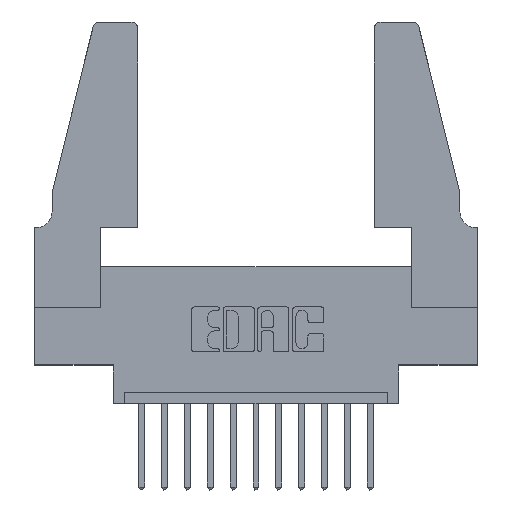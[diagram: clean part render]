
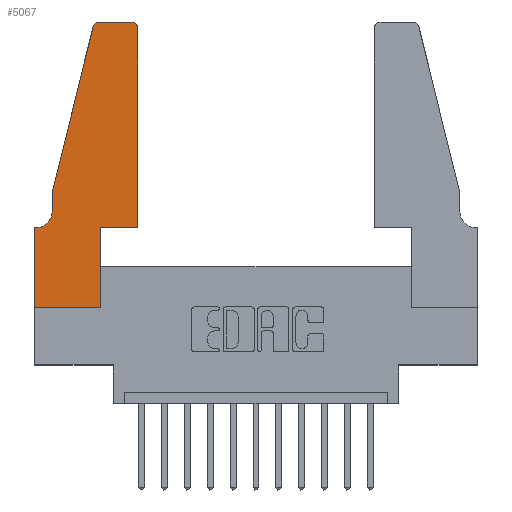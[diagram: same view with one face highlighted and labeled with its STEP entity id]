
A CAD part, top view. The second image highlights one B-rep face of the part: STEP entity #5067.
In plain terms, the highlighted planar face has unit normal (0, 0, 1).
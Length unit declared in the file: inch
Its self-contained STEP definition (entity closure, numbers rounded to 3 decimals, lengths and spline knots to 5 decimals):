
#34 = VECTOR ( 'NONE', #3264, 39.37008 ) ;
#420 = CARTESIAN_POINT ( 'NONE',  ( 0., 0., 0.37 ) ) ;
#542 = ORIENTED_EDGE ( 'NONE', *, *, #3959, .T. ) ;
#629 = EDGE_CURVE ( 'NONE', #13046, #2088, #10502, .T. ) ;
#829 = VERTEX_POINT ( 'NONE', #1325 ) ;
#902 = CARTESIAN_POINT ( 'NONE',  ( 0.0755, 0.5, 0.37 ) ) ;
#965 = VERTEX_POINT ( 'NONE', #14064 ) ;
#1089 = CARTESIAN_POINT ( 'NONE',  ( 0., 0., 0.37 ) ) ;
#1143 = EDGE_CURVE ( 'NONE', #6330, #13046, #6183, .T. ) ;
#1325 = CARTESIAN_POINT ( 'NONE',  ( 0.25487, 1.22718, 0.37 ) ) ;
#1326 = ORIENTED_EDGE ( 'NONE', *, *, #11895, .T. ) ;
#1648 = AXIS2_PLACEMENT_3D ( 'NONE', #6249, #11892, #1726 ) ;
#1726 = DIRECTION ( 'NONE',  ( -1., 0., 0. ) ) ;
#1731 = LINE ( 'NONE', #6070, #8879 ) ;
#2072 = CARTESIAN_POINT ( 'NONE',  ( 0.2605, 1.25, 0.37 ) ) ;
#2088 = VERTEX_POINT ( 'NONE', #2340 ) ;
#2204 = CARTESIAN_POINT ( 'NONE',  ( 0.0755, 0.42, 0.37 ) ) ;
#2340 = CARTESIAN_POINT ( 'NONE',  ( 0.4205, 1.25, 0.37 ) ) ;
#2369 = VERTEX_POINT ( 'NONE', #6469 ) ;
#2382 = CARTESIAN_POINT ( 'NONE',  ( 0.2865, 0.35, 0.37 ) ) ;
#2423 = AXIS2_PLACEMENT_3D ( 'NONE', #4154, #11025, #9827 ) ;
#2503 = DIRECTION ( 'NONE',  ( 1., 0., 0. ) ) ;
#2597 = VERTEX_POINT ( 'NONE', #1089 ) ;
#2632 = VECTOR ( 'NONE', #4961, 39.37008 ) ;
#2845 = LINE ( 'NONE', #13261, #5711 ) ;
#3201 = VERTEX_POINT ( 'NONE', #2204 ) ;
#3264 = DIRECTION ( 'NONE',  ( -1., 0., 0. ) ) ;
#3349 = LINE ( 'NONE', #11802, #2632 ) ;
#3761 = CARTESIAN_POINT ( 'NONE',  ( 0.284, 1.25, 0.37 ) ) ;
#3833 = CARTESIAN_POINT ( 'NONE',  ( 0.4505, 0.35, 0.37 ) ) ;
#3959 = EDGE_CURVE ( 'NONE', #4218, #829, #13787, .T. ) ;
#4154 = CARTESIAN_POINT ( 'NONE',  ( 0.284, 1.22, 0.37 ) ) ;
#4175 = ORIENTED_EDGE ( 'NONE', *, *, #4557, .T. ) ;
#4218 = VERTEX_POINT ( 'NONE', #3761 ) ;
#4557 = EDGE_CURVE ( 'NONE', #2088, #4218, #14088, .T. ) ;
#4961 = DIRECTION ( 'NONE',  ( 0., -1., 0. ) ) ;
#5033 = CARTESIAN_POINT ( 'NONE',  ( 0.0055, 0.35, 0.37 ) ) ;
#5067 = ADVANCED_FACE ( 'NONE', ( #14656 ), #7492, .T. ) ;
#5160 = CARTESIAN_POINT ( 'NONE',  ( 0.4505, 0.35, 0.37 ) ) ;
#5238 = ORIENTED_EDGE ( 'NONE', *, *, #11474, .T. ) ;
#5264 = DIRECTION ( 'NONE',  ( 0., 1., 0. ) ) ;
#5276 = CARTESIAN_POINT ( 'NONE',  ( 0.0755, 0.35, 0.37 ) ) ;
#5323 = DIRECTION ( 'NONE',  ( 0., 0., 1. ) ) ;
#5373 = DIRECTION ( 'NONE',  ( 0., 0., 1. ) ) ;
#5395 = DIRECTION ( 'NONE',  ( -0.239, -0.971, 0. ) ) ;
#5710 = EDGE_CURVE ( 'NONE', #2369, #6330, #2845, .T. ) ;
#5711 = VECTOR ( 'NONE', #14506, 39.37008 ) ;
#6070 = CARTESIAN_POINT ( 'NONE',  ( 0.0755, 0.5, 0.37 ) ) ;
#6183 = LINE ( 'NONE', #5160, #6555 ) ;
#6216 = LINE ( 'NONE', #2382, #13723 ) ;
#6249 = CARTESIAN_POINT ( 'NONE',  ( 0.0055, 0.42, 0.37 ) ) ;
#6330 = VERTEX_POINT ( 'NONE', #3833 ) ;
#6361 = VERTEX_POINT ( 'NONE', #5033 ) ;
#6469 = CARTESIAN_POINT ( 'NONE',  ( 0.2865, 0.35, 0.37 ) ) ;
#6555 = VECTOR ( 'NONE', #5264, 39.37008 ) ;
#6566 = CARTESIAN_POINT ( 'NONE',  ( 0., 0.35, 0.37 ) ) ;
#6747 = EDGE_CURVE ( 'NONE', #965, #2597, #3349, .T. ) ;
#7492 = PLANE ( 'NONE',  #10769 ) ;
#7636 = LINE ( 'NONE', #420, #13898 ) ;
#8405 = ORIENTED_EDGE ( 'NONE', *, *, #14514, .T. ) ;
#8501 = ORIENTED_EDGE ( 'NONE', *, *, #12068, .T. ) ;
#8604 = LINE ( 'NONE', #14433, #10419 ) ;
#8879 = VECTOR ( 'NONE', #13994, 39.37008 ) ;
#9179 = AXIS2_PLACEMENT_3D ( 'NONE', #14462, #5373, #13362 ) ;
#9387 = EDGE_LOOP ( 'NONE', ( #4175, #542, #11279, #14276, #8501, #8405, #9966, #5238, #1326, #11409, #11977, #14247 ) ) ;
#9827 = DIRECTION ( 'NONE',  ( 1., 0., 0. ) ) ;
#9966 = ORIENTED_EDGE ( 'NONE', *, *, #6747, .T. ) ;
#10418 = EDGE_CURVE ( 'NONE', #829, #12775, #8604, .T. ) ;
#10419 = VECTOR ( 'NONE', #5395, 39.37008 ) ;
#10502 = CIRCLE ( 'NONE', #9179, 0.03 ) ;
#10769 = AXIS2_PLACEMENT_3D ( 'NONE', #6566, #5323, #13315 ) ;
#11025 = DIRECTION ( 'NONE',  ( 0., 0., 1. ) ) ;
#11051 = CIRCLE ( 'NONE', #1648, 0.07 ) ;
#11279 = ORIENTED_EDGE ( 'NONE', *, *, #10418, .T. ) ;
#11409 = ORIENTED_EDGE ( 'NONE', *, *, #5710, .T. ) ;
#11474 = EDGE_CURVE ( 'NONE', #2597, #11628, #7636, .T. ) ;
#11628 = VERTEX_POINT ( 'NONE', #11872 ) ;
#11802 = CARTESIAN_POINT ( 'NONE',  ( 0., 0., 0.37 ) ) ;
#11872 = CARTESIAN_POINT ( 'NONE',  ( 0.2865, 0., 0.37 ) ) ;
#11892 = DIRECTION ( 'NONE',  ( 0., 0., -1. ) ) ;
#11895 = EDGE_CURVE ( 'NONE', #11628, #2369, #6216, .T. ) ;
#11977 = ORIENTED_EDGE ( 'NONE', *, *, #1143, .T. ) ;
#12068 = EDGE_CURVE ( 'NONE', #3201, #6361, #11051, .T. ) ;
#12562 = VECTOR ( 'NONE', #14551, 39.37008 ) ;
#12565 = DIRECTION ( 'NONE',  ( 0., 1., 0. ) ) ;
#12571 = EDGE_CURVE ( 'NONE', #12775, #3201, #1731, .T. ) ;
#12775 = VERTEX_POINT ( 'NONE', #902 ) ;
#12826 = CARTESIAN_POINT ( 'NONE',  ( 0.4505, 1.22, 0.37 ) ) ;
#13046 = VERTEX_POINT ( 'NONE', #12826 ) ;
#13261 = CARTESIAN_POINT ( 'NONE',  ( 0.4505, 0.35, 0.37 ) ) ;
#13315 = DIRECTION ( 'NONE',  ( 1., 0., 0. ) ) ;
#13362 = DIRECTION ( 'NONE',  ( 1., 0., 0. ) ) ;
#13723 = VECTOR ( 'NONE', #12565, 39.37008 ) ;
#13787 = CIRCLE ( 'NONE', #2423, 0.03 ) ;
#13812 = LINE ( 'NONE', #5276, #12562 ) ;
#13898 = VECTOR ( 'NONE', #2503, 39.37008 ) ;
#13994 = DIRECTION ( 'NONE',  ( 0., -1., 0. ) ) ;
#14064 = CARTESIAN_POINT ( 'NONE',  ( 0., 0.35, 0.37 ) ) ;
#14088 = LINE ( 'NONE', #2072, #34 ) ;
#14247 = ORIENTED_EDGE ( 'NONE', *, *, #629, .T. ) ;
#14276 = ORIENTED_EDGE ( 'NONE', *, *, #12571, .T. ) ;
#14433 = CARTESIAN_POINT ( 'NONE',  ( 0.0755, 0.5, 0.37 ) ) ;
#14462 = CARTESIAN_POINT ( 'NONE',  ( 0.4205, 1.22, 0.37 ) ) ;
#14506 = DIRECTION ( 'NONE',  ( 1., 0., 0. ) ) ;
#14514 = EDGE_CURVE ( 'NONE', #6361, #965, #13812, .T. ) ;
#14551 = DIRECTION ( 'NONE',  ( -1., 0., 0. ) ) ;
#14656 = FACE_OUTER_BOUND ( 'NONE', #9387, .T. ) ;
